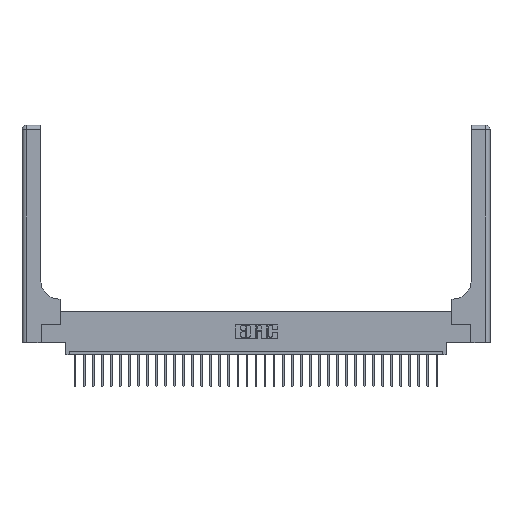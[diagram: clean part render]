
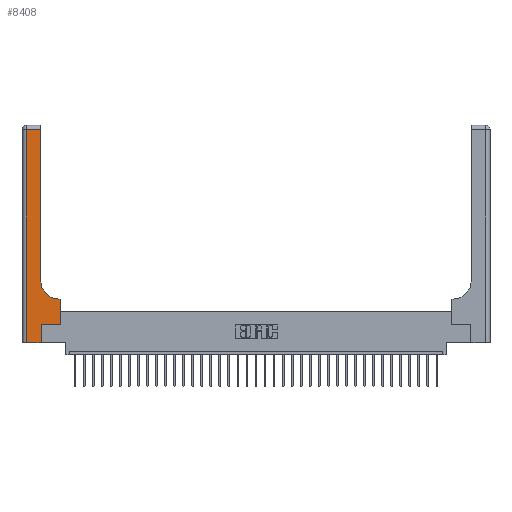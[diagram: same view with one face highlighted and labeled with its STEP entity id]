
A CAD part, top view. The second image highlights one B-rep face of the part: STEP entity #8408.
In plain terms, the highlighted planar face has unit normal (0, 0, 1).
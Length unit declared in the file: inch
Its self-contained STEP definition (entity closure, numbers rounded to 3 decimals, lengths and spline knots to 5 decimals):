
#820 = LINE ( 'NONE', #17933, #1581 ) ;
#1121 = DIRECTION ( 'NONE',  ( 1., 0., 0. ) ) ;
#1581 = VECTOR ( 'NONE', #27492, 39.37008 ) ;
#1785 = PLANE ( 'NONE',  #30758 ) ;
#1858 = CARTESIAN_POINT ( 'NONE',  ( 0.26, 0.85, 0.37 ) ) ;
#2188 = VECTOR ( 'NONE', #28356, 39.37008 ) ;
#2685 = CARTESIAN_POINT ( 'NONE',  ( 0.265, 0., 0.37 ) ) ;
#2778 = VERTEX_POINT ( 'NONE', #7083 ) ;
#2959 = LINE ( 'NONE', #3584, #10418 ) ;
#3109 = VERTEX_POINT ( 'NONE', #1858 ) ;
#3336 = FACE_OUTER_BOUND ( 'NONE', #25791, .T. ) ;
#3584 = CARTESIAN_POINT ( 'NONE',  ( 0.265, 0., 0.37 ) ) ;
#3938 = VERTEX_POINT ( 'NONE', #25300 ) ;
#4124 = VERTEX_POINT ( 'NONE', #2685 ) ;
#4224 = CARTESIAN_POINT ( 'NONE',  ( 0.528, 0.25, 0.37 ) ) ;
#4439 = ORIENTED_EDGE ( 'NONE', *, *, #7294, .T. ) ;
#4773 = VERTEX_POINT ( 'NONE', #13985 ) ;
#5075 = LINE ( 'NONE', #5546, #27845 ) ;
#5140 = ORIENTED_EDGE ( 'NONE', *, *, #7288, .T. ) ;
#5312 = CARTESIAN_POINT ( 'NONE',  ( 0.26, 2.94, 0.37 ) ) ;
#5546 = CARTESIAN_POINT ( 'NONE',  ( 0., 0., 0.37 ) ) ;
#5640 = VECTOR ( 'NONE', #21735, 39.37008 ) ;
#5782 = VECTOR ( 'NONE', #23518, 39.37008 ) ;
#6793 = CARTESIAN_POINT ( 'NONE',  ( 0.06, 3., 0.37 ) ) ;
#6855 = CARTESIAN_POINT ( 'NONE',  ( 0.528, 0.6, 0.37 ) ) ;
#7023 = ORIENTED_EDGE ( 'NONE', *, *, #22423, .T. ) ;
#7083 = CARTESIAN_POINT ( 'NONE',  ( 0.265, 0.25, 0.37 ) ) ;
#7288 = EDGE_CURVE ( 'NONE', #2778, #16757, #20221, .T. ) ;
#7294 = EDGE_CURVE ( 'NONE', #3109, #24755, #11999, .T. ) ;
#7309 = DIRECTION ( 'NONE',  ( 1., 0., 0. ) ) ;
#7468 = VECTOR ( 'NONE', #7309, 39.37008 ) ;
#8408 = ADVANCED_FACE ( 'NONE', ( #3336 ), #1785, .F. ) ;
#8896 = ORIENTED_EDGE ( 'NONE', *, *, #30747, .T. ) ;
#9443 = CARTESIAN_POINT ( 'NONE',  ( 0.528, 0.25, 0.37 ) ) ;
#9479 = LINE ( 'NONE', #6793, #5782 ) ;
#9751 = ORIENTED_EDGE ( 'NONE', *, *, #18140, .T. ) ;
#10418 = VECTOR ( 'NONE', #13415, 39.37008 ) ;
#11482 = EDGE_CURVE ( 'NONE', #24755, #4773, #12296, .T. ) ;
#11967 = ORIENTED_EDGE ( 'NONE', *, *, #21353, .T. ) ;
#11999 = LINE ( 'NONE', #23935, #5640 ) ;
#12296 = LINE ( 'NONE', #26304, #2188 ) ;
#12976 = DIRECTION ( 'NONE',  ( 1., 0., 0. ) ) ;
#13415 = DIRECTION ( 'NONE',  ( 0., 1., 0. ) ) ;
#13985 = CARTESIAN_POINT ( 'NONE',  ( 0.06, 2.94, 0.37 ) ) ;
#15478 = CARTESIAN_POINT ( 'NONE',  ( 0.51, 0.85, 0.37 ) ) ;
#16756 = ORIENTED_EDGE ( 'NONE', *, *, #11482, .T. ) ;
#16757 = VERTEX_POINT ( 'NONE', #9443 ) ;
#17933 = CARTESIAN_POINT ( 'NONE',  ( 0.26, 0.6, 0.37 ) ) ;
#18121 = ORIENTED_EDGE ( 'NONE', *, *, #27232, .T. ) ;
#18140 = EDGE_CURVE ( 'NONE', #16757, #20810, #27710, .T. ) ;
#18294 = DIRECTION ( 'NONE',  ( 0., 0., -1. ) ) ;
#18599 = CIRCLE ( 'NONE', #25190, 0.25 ) ;
#18861 = VERTEX_POINT ( 'NONE', #25800 ) ;
#20221 = LINE ( 'NONE', #26345, #7468 ) ;
#20810 = VERTEX_POINT ( 'NONE', #6855 ) ;
#20929 = DIRECTION ( 'NONE',  ( -1., 0., 0. ) ) ;
#21353 = EDGE_CURVE ( 'NONE', #18861, #3109, #18599, .T. ) ;
#21735 = DIRECTION ( 'NONE',  ( 0., 1., 0. ) ) ;
#22423 = EDGE_CURVE ( 'NONE', #20810, #18861, #820, .T. ) ;
#22901 = DIRECTION ( 'NONE',  ( 0., 0., -1. ) ) ;
#23005 = CARTESIAN_POINT ( 'NONE',  ( 0., 3., 0.37 ) ) ;
#23216 = DIRECTION ( 'NONE',  ( 0., 1., 0. ) ) ;
#23518 = DIRECTION ( 'NONE',  ( 0., -1., 0. ) ) ;
#23935 = CARTESIAN_POINT ( 'NONE',  ( 0.26, 3., 0.37 ) ) ;
#24019 = VECTOR ( 'NONE', #23216, 39.37008 ) ;
#24755 = VERTEX_POINT ( 'NONE', #5312 ) ;
#25190 = AXIS2_PLACEMENT_3D ( 'NONE', #15478, #18294, #1121 ) ;
#25300 = CARTESIAN_POINT ( 'NONE',  ( 0.06, 0., 0.37 ) ) ;
#25791 = EDGE_LOOP ( 'NONE', ( #4439, #16756, #18121, #8896, #28704, #5140, #9751, #7023, #11967 ) ) ;
#25800 = CARTESIAN_POINT ( 'NONE',  ( 0.51, 0.6, 0.37 ) ) ;
#26304 = CARTESIAN_POINT ( 'NONE',  ( 0., 2.94, 0.37 ) ) ;
#26345 = CARTESIAN_POINT ( 'NONE',  ( 0.265, 0.25, 0.37 ) ) ;
#27232 = EDGE_CURVE ( 'NONE', #4773, #3938, #9479, .T. ) ;
#27492 = DIRECTION ( 'NONE',  ( -1., 0., 0. ) ) ;
#27710 = LINE ( 'NONE', #4224, #24019 ) ;
#27845 = VECTOR ( 'NONE', #12976, 39.37008 ) ;
#28356 = DIRECTION ( 'NONE',  ( -1., 0., 0. ) ) ;
#28598 = EDGE_CURVE ( 'NONE', #4124, #2778, #2959, .T. ) ;
#28704 = ORIENTED_EDGE ( 'NONE', *, *, #28598, .T. ) ;
#30747 = EDGE_CURVE ( 'NONE', #3938, #4124, #5075, .T. ) ;
#30758 = AXIS2_PLACEMENT_3D ( 'NONE', #23005, #22901, #20929 ) ;
